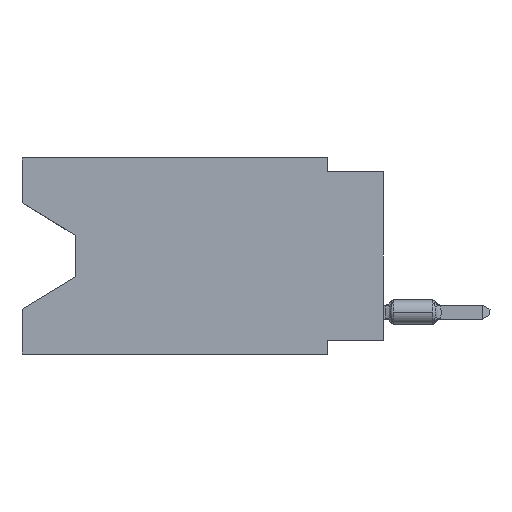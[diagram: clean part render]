
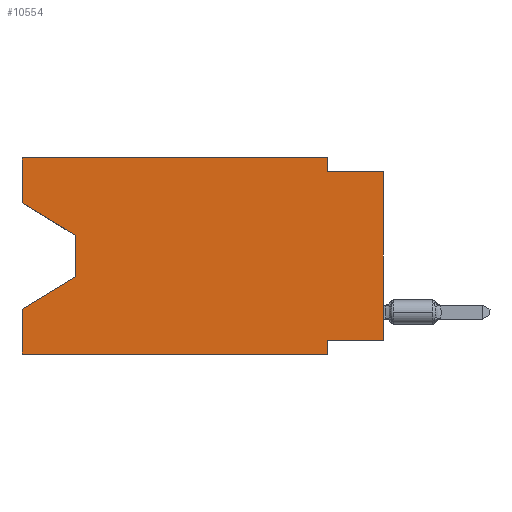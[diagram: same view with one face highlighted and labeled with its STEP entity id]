
A CAD part, left-side view. The second image highlights one B-rep face of the part: STEP entity #10554.
In plain terms, the highlighted planar face has unit normal (-1, 0, 0).
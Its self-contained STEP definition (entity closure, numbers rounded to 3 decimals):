
#215 = VECTOR ( 'NONE', #7195, 1000. ) ;
#353 = CARTESIAN_POINT ( 'NONE',  ( 0., 16.383, 0. ) ) ;
#404 = CARTESIAN_POINT ( 'NONE',  ( 0., 2.54, -8.255 ) ) ;
#560 = ORIENTED_EDGE ( 'NONE', *, *, #14429, .F. ) ;
#650 = VERTEX_POINT ( 'NONE', #14021 ) ;
#1086 = EDGE_CURVE ( 'NONE', #6457, #15827, #12755, .T. ) ;
#1098 = CARTESIAN_POINT ( 'NONE',  ( 0., 16.383, 0. ) ) ;
#1191 = DIRECTION ( 'NONE',  ( 0., -1., 0. ) ) ;
#1263 = DIRECTION ( 'NONE',  ( 0., -0.855, -0.519 ) ) ;
#1357 = VERTEX_POINT ( 'NONE', #13789 ) ;
#1407 = ORIENTED_EDGE ( 'NONE', *, *, #3930, .T. ) ;
#1470 = LINE ( 'NONE', #12888, #7380 ) ;
#1499 = EDGE_CURVE ( 'NONE', #12405, #15827, #1470, .T. ) ;
#2118 = ORIENTED_EDGE ( 'NONE', *, *, #1086, .T. ) ;
#2436 = CARTESIAN_POINT ( 'NONE',  ( 0., 13.97, -3.505 ) ) ;
#2860 = FACE_OUTER_BOUND ( 'NONE', #3190, .T. ) ;
#2983 = CARTESIAN_POINT ( 'NONE',  ( 0., 0., -8.255 ) ) ;
#3129 = LINE ( 'NONE', #14857, #6364 ) ;
#3153 = EDGE_CURVE ( 'NONE', #11844, #12405, #15883, .T. ) ;
#3190 = EDGE_LOOP ( 'NONE', ( #14980, #10893, #1407, #12175, #2118, #13909, #11689, #15665, #15053, #12033, #560, #16537 ) ) ;
#3449 = CARTESIAN_POINT ( 'NONE',  ( 0., 0., -0.635 ) ) ;
#3667 = VECTOR ( 'NONE', #1263, 1000. ) ;
#3930 = EDGE_CURVE ( 'NONE', #650, #1357, #8291, .T. ) ;
#3992 = DIRECTION ( 'NONE',  ( 0., 0., -1. ) ) ;
#4294 = DIRECTION ( 'NONE',  ( 0., 0., -1. ) ) ;
#4459 = DIRECTION ( 'NONE',  ( 0., 0., 1. ) ) ;
#4784 = VERTEX_POINT ( 'NONE', #11102 ) ;
#4848 = LINE ( 'NONE', #9967, #13422 ) ;
#5007 = VECTOR ( 'NONE', #15012, 1000. ) ;
#5177 = VERTEX_POINT ( 'NONE', #11086 ) ;
#5465 = DIRECTION ( 'NONE',  ( 0., 0., -1. ) ) ;
#5937 = VERTEX_POINT ( 'NONE', #6868 ) ;
#6053 = CARTESIAN_POINT ( 'NONE',  ( 0., 2.54, 0. ) ) ;
#6102 = VECTOR ( 'NONE', #10863, 1000. ) ;
#6298 = DIRECTION ( 'NONE',  ( 0., 0., 1. ) ) ;
#6364 = VECTOR ( 'NONE', #4459, 1000. ) ;
#6457 = VERTEX_POINT ( 'NONE', #12134 ) ;
#6540 = CARTESIAN_POINT ( 'NONE',  ( 0., 16.383, -2.038 ) ) ;
#6868 = CARTESIAN_POINT ( 'NONE',  ( 0., 16.383, 0. ) ) ;
#7083 = LINE ( 'NONE', #12196, #6102 ) ;
#7195 = DIRECTION ( 'NONE',  ( 0., 0.855, -0.519 ) ) ;
#7380 = VECTOR ( 'NONE', #3992, 1000. ) ;
#7386 = CARTESIAN_POINT ( 'NONE',  ( 0., 16.383, -8.89 ) ) ;
#7554 = LINE ( 'NONE', #6540, #3667 ) ;
#8291 = LINE ( 'NONE', #10981, #215 ) ;
#8380 = CARTESIAN_POINT ( 'NONE',  ( 0., 0., -8.255 ) ) ;
#8449 = VECTOR ( 'NONE', #1191, 1000. ) ;
#8474 = EDGE_CURVE ( 'NONE', #14644, #650, #16342, .T. ) ;
#9160 = DIRECTION ( 'NONE',  ( 1., 0., 0. ) ) ;
#9178 = EDGE_CURVE ( 'NONE', #11844, #12736, #7083, .T. ) ;
#9500 = LINE ( 'NONE', #10597, #13304 ) ;
#9575 = VECTOR ( 'NONE', #13452, 1000. ) ;
#9662 = CARTESIAN_POINT ( 'NONE',  ( 0., 2.54, -8.89 ) ) ;
#9701 = LINE ( 'NONE', #14872, #13695 ) ;
#9967 = CARTESIAN_POINT ( 'NONE',  ( 0., 0., -0.635 ) ) ;
#10554 = ADVANCED_FACE ( 'NONE', ( #2860 ), #15523, .F. ) ;
#10597 = CARTESIAN_POINT ( 'NONE',  ( 0., 2.54, 0. ) ) ;
#10863 = DIRECTION ( 'NONE',  ( 0., 0., 1. ) ) ;
#10893 = ORIENTED_EDGE ( 'NONE', *, *, #8474, .T. ) ;
#10958 = DIRECTION ( 'NONE',  ( 0., -1., 0. ) ) ;
#10981 = CARTESIAN_POINT ( 'NONE',  ( 0., 13.97, -5.385 ) ) ;
#11086 = CARTESIAN_POINT ( 'NONE',  ( 0., 16.383, -2.038 ) ) ;
#11102 = CARTESIAN_POINT ( 'NONE',  ( 0., 2.54, -0.635 ) ) ;
#11689 = ORIENTED_EDGE ( 'NONE', *, *, #3153, .F. ) ;
#11844 = VERTEX_POINT ( 'NONE', #8380 ) ;
#11955 = EDGE_CURVE ( 'NONE', #4784, #12736, #4848, .T. ) ;
#12033 = ORIENTED_EDGE ( 'NONE', *, *, #13048, .F. ) ;
#12057 = EDGE_CURVE ( 'NONE', #6457, #1357, #16509, .T. ) ;
#12134 = CARTESIAN_POINT ( 'NONE',  ( 0., 16.383, -8.89 ) ) ;
#12175 = ORIENTED_EDGE ( 'NONE', *, *, #12057, .F. ) ;
#12196 = CARTESIAN_POINT ( 'NONE',  ( 0., 0., 0. ) ) ;
#12405 = VERTEX_POINT ( 'NONE', #404 ) ;
#12564 = DIRECTION ( 'NONE',  ( 0., -1., 0. ) ) ;
#12736 = VERTEX_POINT ( 'NONE', #3449 ) ;
#12755 = LINE ( 'NONE', #7386, #8449 ) ;
#12888 = CARTESIAN_POINT ( 'NONE',  ( 0., 2.54, -8.89 ) ) ;
#12893 = EDGE_CURVE ( 'NONE', #5177, #14644, #7554, .T. ) ;
#13013 = VECTOR ( 'NONE', #6298, 1000. ) ;
#13048 = EDGE_CURVE ( 'NONE', #15350, #4784, #9500, .T. ) ;
#13304 = VECTOR ( 'NONE', #4294, 1000. ) ;
#13410 = EDGE_CURVE ( 'NONE', #5177, #5937, #3129, .T. ) ;
#13422 = VECTOR ( 'NONE', #12564, 1000. ) ;
#13452 = DIRECTION ( 'NONE',  ( 0., 1., 0. ) ) ;
#13695 = VECTOR ( 'NONE', #10958, 1000. ) ;
#13789 = CARTESIAN_POINT ( 'NONE',  ( 0., 16.383, -6.852 ) ) ;
#13909 = ORIENTED_EDGE ( 'NONE', *, *, #1499, .F. ) ;
#14021 = CARTESIAN_POINT ( 'NONE',  ( 0., 13.97, -5.385 ) ) ;
#14429 = EDGE_CURVE ( 'NONE', #5937, #15350, #9701, .T. ) ;
#14493 = AXIS2_PLACEMENT_3D ( 'NONE', #353, #9160, #5465 ) ;
#14644 = VERTEX_POINT ( 'NONE', #16291 ) ;
#14857 = CARTESIAN_POINT ( 'NONE',  ( 0., 16.383, 0. ) ) ;
#14872 = CARTESIAN_POINT ( 'NONE',  ( 0., 16.383, 0. ) ) ;
#14980 = ORIENTED_EDGE ( 'NONE', *, *, #12893, .T. ) ;
#15012 = DIRECTION ( 'NONE',  ( 0., 0., -1. ) ) ;
#15053 = ORIENTED_EDGE ( 'NONE', *, *, #11955, .F. ) ;
#15350 = VERTEX_POINT ( 'NONE', #6053 ) ;
#15523 = PLANE ( 'NONE',  #14493 ) ;
#15665 = ORIENTED_EDGE ( 'NONE', *, *, #9178, .T. ) ;
#15827 = VERTEX_POINT ( 'NONE', #9662 ) ;
#15883 = LINE ( 'NONE', #2983, #9575 ) ;
#16291 = CARTESIAN_POINT ( 'NONE',  ( 0., 13.97, -3.505 ) ) ;
#16342 = LINE ( 'NONE', #2436, #5007 ) ;
#16509 = LINE ( 'NONE', #1098, #13013 ) ;
#16537 = ORIENTED_EDGE ( 'NONE', *, *, #13410, .F. ) ;
